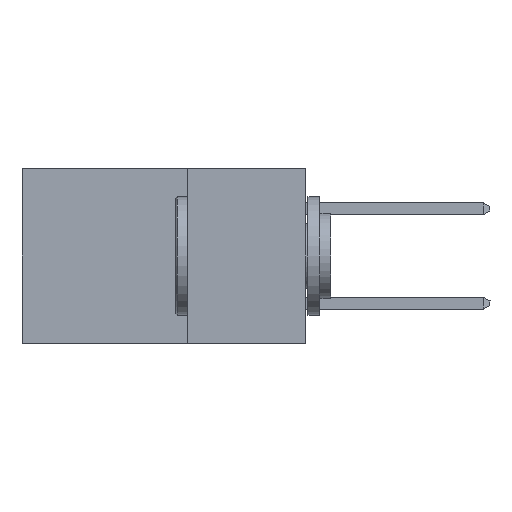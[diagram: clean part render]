
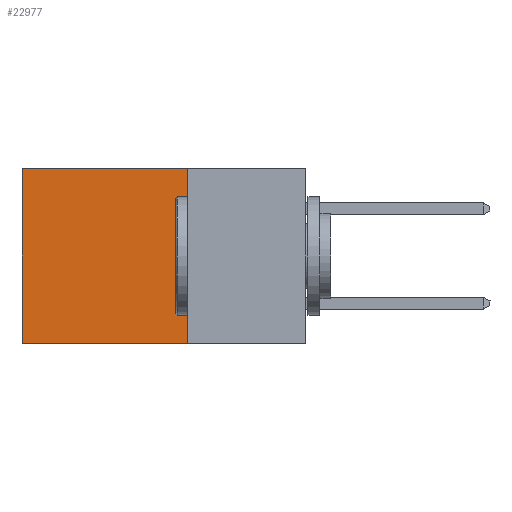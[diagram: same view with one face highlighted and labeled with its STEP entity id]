
A CAD part, left-side view. The second image highlights one B-rep face of the part: STEP entity #22977.
In plain terms, the highlighted planar face has unit normal (-1, 0, 0).
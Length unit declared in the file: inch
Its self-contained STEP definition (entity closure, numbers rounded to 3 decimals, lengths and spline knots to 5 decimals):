
#2745 = ORIENTED_EDGE ( 'NONE', *, *, #19533, .F. ) ;
#2805 = VERTEX_POINT ( 'NONE', #14343 ) ;
#3648 = AXIS2_PLACEMENT_3D ( 'NONE', #30595, #9659, #23031 ) ;
#4516 = EDGE_LOOP ( 'NONE', ( #31262, #2745, #32713, #5558 ) ) ;
#4535 = DIRECTION ( 'NONE',  ( 0., 0., -1. ) ) ;
#4769 = CARTESIAN_POINT ( 'NONE',  ( 0.298, 0.6, 0. ) ) ;
#4842 = FACE_OUTER_BOUND ( 'NONE', #4516, .T. ) ;
#4848 = VERTEX_POINT ( 'NONE', #17117 ) ;
#5558 = ORIENTED_EDGE ( 'NONE', *, *, #30454, .T. ) ;
#5599 = CARTESIAN_POINT ( 'NONE',  ( 0.298, 0.25, -0.37 ) ) ;
#6698 = VECTOR ( 'NONE', #20130, 39.37008 ) ;
#6723 = EDGE_CURVE ( 'NONE', #2805, #12580, #25725, .T. ) ;
#7394 = CARTESIAN_POINT ( 'NONE',  ( 0.298, 0.6, -0.37 ) ) ;
#7777 = VECTOR ( 'NONE', #4535, 39.37008 ) ;
#8436 = CARTESIAN_POINT ( 'NONE',  ( 0.298, 0.25, 0. ) ) ;
#9659 = DIRECTION ( 'NONE',  ( 1., 0., 0. ) ) ;
#10621 = LINE ( 'NONE', #17525, #27782 ) ;
#12580 = VERTEX_POINT ( 'NONE', #7394 ) ;
#12692 = DIRECTION ( 'NONE',  ( 0., 0., -1. ) ) ;
#14343 = CARTESIAN_POINT ( 'NONE',  ( 0.298, 0.6, 0. ) ) ;
#17117 = CARTESIAN_POINT ( 'NONE',  ( 0.298, 0.25, -0.37 ) ) ;
#17525 = CARTESIAN_POINT ( 'NONE',  ( 0.298, 0.25, 0. ) ) ;
#19533 = EDGE_CURVE ( 'NONE', #4848, #12580, #21355, .T. ) ;
#20130 = DIRECTION ( 'NONE',  ( 0., 1., 0. ) ) ;
#21355 = LINE ( 'NONE', #5599, #6698 ) ;
#21725 = LINE ( 'NONE', #23091, #32007 ) ;
#22977 = ADVANCED_FACE ( 'NONE', ( #4842 ), #33462, .F. ) ;
#23031 = DIRECTION ( 'NONE',  ( 0., 0., -1. ) ) ;
#23091 = CARTESIAN_POINT ( 'NONE',  ( 0.298, 0.25, 0. ) ) ;
#24048 = VERTEX_POINT ( 'NONE', #8436 ) ;
#25725 = LINE ( 'NONE', #4769, #7777 ) ;
#25935 = DIRECTION ( 'NONE',  ( 0., 1., 0. ) ) ;
#26014 = EDGE_CURVE ( 'NONE', #24048, #4848, #10621, .T. ) ;
#27782 = VECTOR ( 'NONE', #12692, 39.37008 ) ;
#30454 = EDGE_CURVE ( 'NONE', #24048, #2805, #21725, .T. ) ;
#30595 = CARTESIAN_POINT ( 'NONE',  ( 0.298, 0.25, 0. ) ) ;
#31262 = ORIENTED_EDGE ( 'NONE', *, *, #6723, .T. ) ;
#32007 = VECTOR ( 'NONE', #25935, 39.37008 ) ;
#32713 = ORIENTED_EDGE ( 'NONE', *, *, #26014, .F. ) ;
#33462 = PLANE ( 'NONE',  #3648 ) ;
